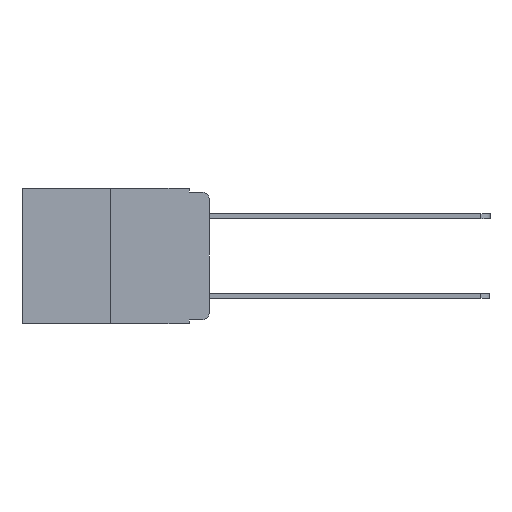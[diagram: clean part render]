
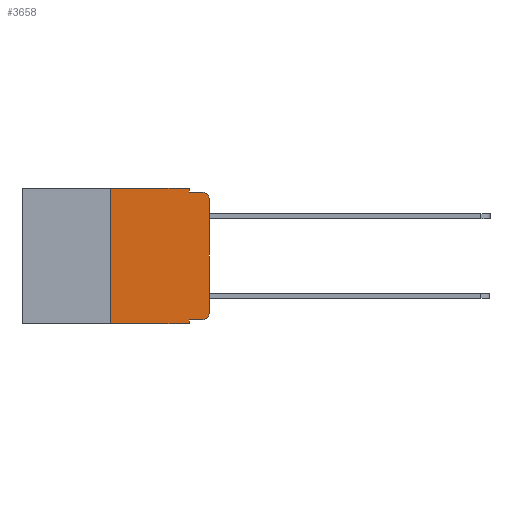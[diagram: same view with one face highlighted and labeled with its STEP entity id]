
A CAD part, left-side view. The second image highlights one B-rep face of the part: STEP entity #3658.
In plain terms, the highlighted planar face has unit normal (-1, 0, 0).
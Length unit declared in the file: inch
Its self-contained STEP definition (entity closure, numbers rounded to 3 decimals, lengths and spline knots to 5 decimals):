
#378 = CARTESIAN_POINT ( 'NONE',  ( 0., 0.25, 0. ) ) ;
#684 = AXIS2_PLACEMENT_3D ( 'NONE', #11092, #2271, #12515 ) ;
#747 = CARTESIAN_POINT ( 'NONE',  ( 0., 0.051, 0. ) ) ;
#1122 = ORIENTED_EDGE ( 'NONE', *, *, #5030, .T. ) ;
#1126 = CARTESIAN_POINT ( 'NONE',  ( 0., 0.051, -0.01 ) ) ;
#1264 = CARTESIAN_POINT ( 'NONE',  ( 0., 0.25, 0. ) ) ;
#1606 = AXIS2_PLACEMENT_3D ( 'NONE', #9753, #11257, #2457 ) ;
#1633 = EDGE_CURVE ( 'NONE', #4181, #10003, #9638, .T. ) ;
#2182 = DIRECTION ( 'NONE',  ( 0., 0., -1. ) ) ;
#2271 = DIRECTION ( 'NONE',  ( -1., 0., 0. ) ) ;
#2457 = DIRECTION ( 'NONE',  ( 0., 0., -1. ) ) ;
#2582 = VECTOR ( 'NONE', #14419, 39.37008 ) ;
#2638 = LINE ( 'NONE', #18164, #10472 ) ;
#2991 = EDGE_CURVE ( 'NONE', #6888, #14240, #10278, .T. ) ;
#3058 = ORIENTED_EDGE ( 'NONE', *, *, #14476, .F. ) ;
#3658 = ADVANCED_FACE ( 'NONE', ( #8009 ), #9814, .F. ) ;
#4181 = VERTEX_POINT ( 'NONE', #6647 ) ;
#4235 = DIRECTION ( 'NONE',  ( 0., -1., 0. ) ) ;
#4376 = DIRECTION ( 'NONE',  ( 0., 0., 1. ) ) ;
#4507 = EDGE_LOOP ( 'NONE', ( #1122, #5672, #17560, #3058, #7482, #18884, #13975, #10645, #7723, #4744 ) ) ;
#4744 = ORIENTED_EDGE ( 'NONE', *, *, #2991, .T. ) ;
#5030 = EDGE_CURVE ( 'NONE', #14240, #13765, #10592, .T. ) ;
#5318 = VECTOR ( 'NONE', #15394, 39.37008 ) ;
#5672 = ORIENTED_EDGE ( 'NONE', *, *, #12805, .T. ) ;
#5863 = CARTESIAN_POINT ( 'NONE',  ( 0., 0., 0. ) ) ;
#5891 = CARTESIAN_POINT ( 'NONE',  ( 0., 0.473, -0.343 ) ) ;
#6229 = VERTEX_POINT ( 'NONE', #378 ) ;
#6537 = LINE ( 'NONE', #1126, #9921 ) ;
#6647 = CARTESIAN_POINT ( 'NONE',  ( 0., 0.051, -0.333 ) ) ;
#6787 = CIRCLE ( 'NONE', #16079, 0.02 ) ;
#6888 = VERTEX_POINT ( 'NONE', #16424 ) ;
#7165 = CARTESIAN_POINT ( 'NONE',  ( 0., 0.02, -0.03 ) ) ;
#7482 = ORIENTED_EDGE ( 'NONE', *, *, #16251, .F. ) ;
#7723 = ORIENTED_EDGE ( 'NONE', *, *, #9494, .T. ) ;
#8009 = FACE_OUTER_BOUND ( 'NONE', #4507, .T. ) ;
#8203 = DIRECTION ( 'NONE',  ( 0., -1., 0. ) ) ;
#8639 = DIRECTION ( 'NONE',  ( 0., 0., -1. ) ) ;
#8665 = VERTEX_POINT ( 'NONE', #9724 ) ;
#8784 = CARTESIAN_POINT ( 'NONE',  ( 0., 0.25, -0.343 ) ) ;
#8826 = LINE ( 'NONE', #5891, #15959 ) ;
#8869 = VERTEX_POINT ( 'NONE', #10147 ) ;
#8887 = VERTEX_POINT ( 'NONE', #8784 ) ;
#9419 = CARTESIAN_POINT ( 'NONE',  ( 0., 0., -0.03 ) ) ;
#9494 = EDGE_CURVE ( 'NONE', #4181, #6888, #10418, .T. ) ;
#9638 = LINE ( 'NONE', #13497, #5318 ) ;
#9724 = CARTESIAN_POINT ( 'NONE',  ( 0., 0.02, -0.01 ) ) ;
#9753 = CARTESIAN_POINT ( 'NONE',  ( 0., 0.473, 0. ) ) ;
#9814 = PLANE ( 'NONE',  #1606 ) ;
#9921 = VECTOR ( 'NONE', #4235, 39.37008 ) ;
#9968 = LINE ( 'NONE', #1264, #13312 ) ;
#10003 = VERTEX_POINT ( 'NONE', #14263 ) ;
#10147 = CARTESIAN_POINT ( 'NONE',  ( 0., 0.051, -0.01 ) ) ;
#10278 = CIRCLE ( 'NONE', #684, 0.02 ) ;
#10418 = LINE ( 'NONE', #12984, #2582 ) ;
#10472 = VECTOR ( 'NONE', #8203, 39.37008 ) ;
#10592 = LINE ( 'NONE', #5863, #17287 ) ;
#10645 = ORIENTED_EDGE ( 'NONE', *, *, #1633, .F. ) ;
#11012 = CARTESIAN_POINT ( 'NONE',  ( 0., 0.051, 0. ) ) ;
#11092 = CARTESIAN_POINT ( 'NONE',  ( 0., 0.02, -0.313 ) ) ;
#11257 = DIRECTION ( 'NONE',  ( 1., 0., 0. ) ) ;
#11446 = LINE ( 'NONE', #11012, #16564 ) ;
#12214 = EDGE_CURVE ( 'NONE', #8887, #6229, #9968, .T. ) ;
#12515 = DIRECTION ( 'NONE',  ( 0., 0., -1. ) ) ;
#12805 = EDGE_CURVE ( 'NONE', #13765, #8665, #6787, .T. ) ;
#12984 = CARTESIAN_POINT ( 'NONE',  ( 0., 0.051, -0.333 ) ) ;
#13312 = VECTOR ( 'NONE', #4376, 39.37008 ) ;
#13313 = VERTEX_POINT ( 'NONE', #747 ) ;
#13497 = CARTESIAN_POINT ( 'NONE',  ( 0., 0.051, 0. ) ) ;
#13765 = VERTEX_POINT ( 'NONE', #9419 ) ;
#13975 = ORIENTED_EDGE ( 'NONE', *, *, #17906, .T. ) ;
#14240 = VERTEX_POINT ( 'NONE', #17513 ) ;
#14263 = CARTESIAN_POINT ( 'NONE',  ( 0., 0.051, -0.343 ) ) ;
#14419 = DIRECTION ( 'NONE',  ( 0., -1., 0. ) ) ;
#14440 = DIRECTION ( 'NONE',  ( 0., 0., 1. ) ) ;
#14476 = EDGE_CURVE ( 'NONE', #13313, #8869, #11446, .T. ) ;
#15394 = DIRECTION ( 'NONE',  ( 0., 0., -1. ) ) ;
#15959 = VECTOR ( 'NONE', #18897, 39.37008 ) ;
#16079 = AXIS2_PLACEMENT_3D ( 'NONE', #7165, #17178, #8639 ) ;
#16251 = EDGE_CURVE ( 'NONE', #6229, #13313, #2638, .T. ) ;
#16424 = CARTESIAN_POINT ( 'NONE',  ( 0., 0.02, -0.333 ) ) ;
#16564 = VECTOR ( 'NONE', #2182, 39.37008 ) ;
#17178 = DIRECTION ( 'NONE',  ( -1., 0., 0. ) ) ;
#17287 = VECTOR ( 'NONE', #14440, 39.37008 ) ;
#17513 = CARTESIAN_POINT ( 'NONE',  ( 0., 0., -0.313 ) ) ;
#17560 = ORIENTED_EDGE ( 'NONE', *, *, #18446, .F. ) ;
#17906 = EDGE_CURVE ( 'NONE', #8887, #10003, #8826, .T. ) ;
#18164 = CARTESIAN_POINT ( 'NONE',  ( 0., 0.473, 0. ) ) ;
#18446 = EDGE_CURVE ( 'NONE', #8869, #8665, #6537, .T. ) ;
#18884 = ORIENTED_EDGE ( 'NONE', *, *, #12214, .F. ) ;
#18897 = DIRECTION ( 'NONE',  ( 0., -1., 0. ) ) ;
